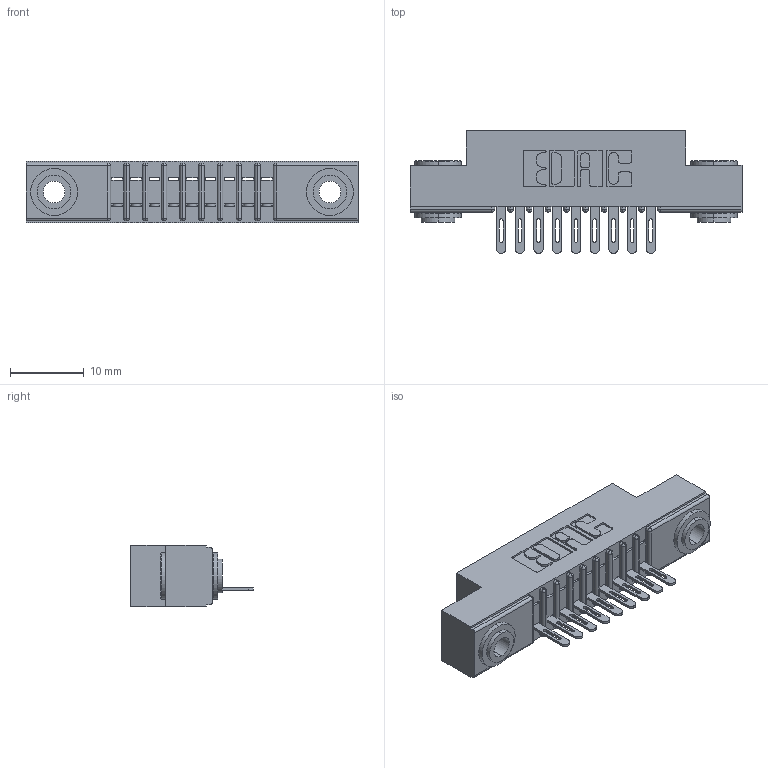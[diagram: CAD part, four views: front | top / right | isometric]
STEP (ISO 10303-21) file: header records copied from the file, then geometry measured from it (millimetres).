
FILE_DESCRIPTION (( 'STEP AP203' ), '1' );
FILE_NAME ('341-009-500-103.STEP', '2019-08-09T16:04:14', ( '' ), ( '' ), 'SwSTEP 2.0', 'SolidWorks 2016', '' );
FILE_SCHEMA (( 'CONFIG_CONTROL_DESIGN' ));
Length unit declared in the file: inch
Products named in the file (4): 341 Part_.156 (3.96) Dia Mounting Holes; 341-009-500-103; 345-250-002_345-250-002-102; 341-292-001_341-292-100
Assembly tree (12 placements, depth 2):
  341-009-500-103
    341 Part_.156 (3.96) Dia Mounting Holes
    341-292-001_341-292-100  x9
    345-250-002_345-250-002-102  x2
Bounding box: 45.09 x 16.69 x 8.38 mm (x, y, z)
Volume: 2550.7 mm3; surface area: 4399.2 mm2
Topology: 12 solids, 12 shells, 906 faces, 2561 edges, 1646 vertices
Faces by surface type: plane 533, cylinder 329, sphere 20, torus 16, cone 8
Entity records: 16073 total; most frequent: CARTESIAN_POINT 2691, ORIENTED_EDGE 2670, DIRECTION 2645, EDGE_CURVE 1335, VECTOR 1029, LINE 1029, VERTEX_POINT 854, AXIS2_PLACEMENT_3D 808
